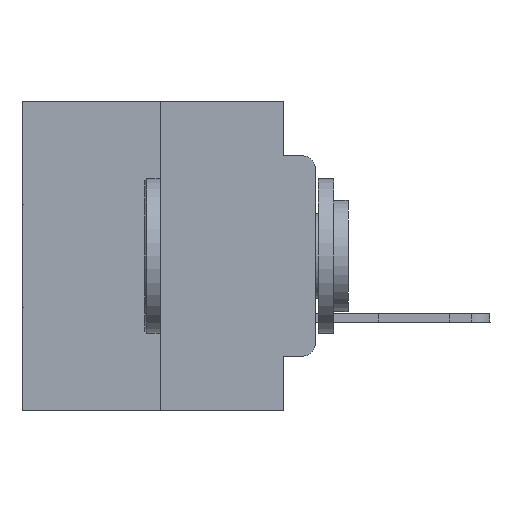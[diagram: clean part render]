
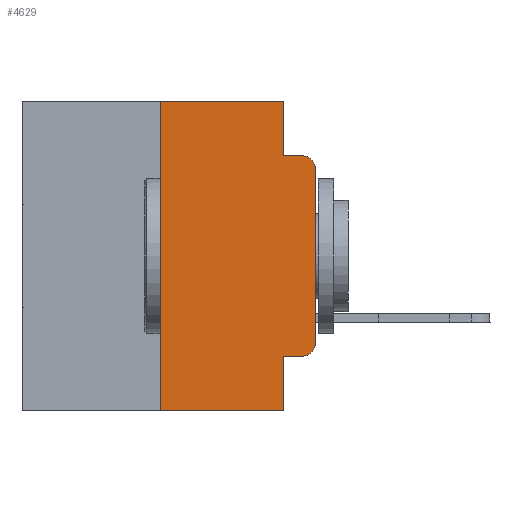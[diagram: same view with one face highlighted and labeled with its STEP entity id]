
A CAD part, left-side view. The second image highlights one B-rep face of the part: STEP entity #4629.
In plain terms, the highlighted planar face has unit normal (-1, 0, 0).
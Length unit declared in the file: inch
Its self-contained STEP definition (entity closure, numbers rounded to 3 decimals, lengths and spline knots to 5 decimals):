
#141 = EDGE_CURVE ( 'NONE', #13487, #4474, #5541, .T. ) ;
#193 = CARTESIAN_POINT ( 'NONE',  ( 0., 0.051, -0.0885 ) ) ;
#568 = CARTESIAN_POINT ( 'NONE',  ( 0., 0.051, 0. ) ) ;
#1051 = CARTESIAN_POINT ( 'NONE',  ( 0., 0.051, -0.4115 ) ) ;
#1135 = FACE_OUTER_BOUND ( 'NONE', #25109, .T. ) ;
#1803 = CARTESIAN_POINT ( 'NONE',  ( 0., 0.051, 0. ) ) ;
#2181 = CARTESIAN_POINT ( 'NONE',  ( 0., 0.02, -0.3915 ) ) ;
#2285 = EDGE_CURVE ( 'NONE', #9579, #4019, #24127, .T. ) ;
#2543 = VECTOR ( 'NONE', #25909, 39.37008 ) ;
#2561 = DIRECTION ( 'NONE',  ( 0., 0., 1. ) ) ;
#2709 = LINE ( 'NONE', #16795, #23457 ) ;
#2901 = DIRECTION ( 'NONE',  ( 0., 0., -1. ) ) ;
#3704 = VERTEX_POINT ( 'NONE', #4943 ) ;
#3713 = VECTOR ( 'NONE', #14315, 39.37008 ) ;
#3853 = CARTESIAN_POINT ( 'NONE',  ( 0., 0.02, -0.1085 ) ) ;
#3874 = CARTESIAN_POINT ( 'NONE',  ( 0., 0.25, -0.5 ) ) ;
#4019 = VERTEX_POINT ( 'NONE', #193 ) ;
#4149 = VERTEX_POINT ( 'NONE', #23626 ) ;
#4474 = VERTEX_POINT ( 'NONE', #25907 ) ;
#4629 = ADVANCED_FACE ( 'NONE', ( #1135 ), #26872, .F. ) ;
#4943 = CARTESIAN_POINT ( 'NONE',  ( 0., 0.051, -0.5 ) ) ;
#5349 = LINE ( 'NONE', #16885, #22020 ) ;
#5541 = LINE ( 'NONE', #1051, #22198 ) ;
#5727 = DIRECTION ( 'NONE',  ( -1., 0., 0. ) ) ;
#6321 = EDGE_CURVE ( 'NONE', #13487, #3704, #18810, .T. ) ;
#6804 = VERTEX_POINT ( 'NONE', #3874 ) ;
#6928 = DIRECTION ( 'NONE',  ( -1., 0., 0. ) ) ;
#7180 = VECTOR ( 'NONE', #21510, 39.37008 ) ;
#8410 = CARTESIAN_POINT ( 'NONE',  ( 0., 0.473, -0.5 ) ) ;
#9579 = VERTEX_POINT ( 'NONE', #568 ) ;
#9618 = LINE ( 'NONE', #27242, #10628 ) ;
#9858 = EDGE_CURVE ( 'NONE', #24876, #9579, #2709, .T. ) ;
#10045 = DIRECTION ( 'NONE',  ( 0., -1., 0. ) ) ;
#10065 = LINE ( 'NONE', #19985, #11460 ) ;
#10079 = AXIS2_PLACEMENT_3D ( 'NONE', #2181, #6928, #13445 ) ;
#10628 = VECTOR ( 'NONE', #18607, 39.37008 ) ;
#11460 = VECTOR ( 'NONE', #2561, 39.37008 ) ;
#11518 = CARTESIAN_POINT ( 'NONE',  ( 0., 0.473, 0. ) ) ;
#12110 = ORIENTED_EDGE ( 'NONE', *, *, #27522, .F. ) ;
#13088 = DIRECTION ( 'NONE',  ( 0., -1., 0. ) ) ;
#13153 = EDGE_CURVE ( 'NONE', #4149, #20485, #19581, .T. ) ;
#13445 = DIRECTION ( 'NONE',  ( 0., 0., -1. ) ) ;
#13487 = VERTEX_POINT ( 'NONE', #20907 ) ;
#14262 = ORIENTED_EDGE ( 'NONE', *, *, #9858, .F. ) ;
#14315 = DIRECTION ( 'NONE',  ( 0., 0., -1. ) ) ;
#14551 = AXIS2_PLACEMENT_3D ( 'NONE', #11518, #24292, #2901 ) ;
#14731 = CARTESIAN_POINT ( 'NONE',  ( 0., 0.02, -0.0885 ) ) ;
#16591 = ORIENTED_EDGE ( 'NONE', *, *, #26675, .T. ) ;
#16795 = CARTESIAN_POINT ( 'NONE',  ( 0., 0.473, 0. ) ) ;
#16858 = CARTESIAN_POINT ( 'NONE',  ( 0., 0.051, 0. ) ) ;
#16885 = CARTESIAN_POINT ( 'NONE',  ( 0., 0., 0. ) ) ;
#17804 = CARTESIAN_POINT ( 'NONE',  ( 0., 0., -0.3915 ) ) ;
#18554 = CARTESIAN_POINT ( 'NONE',  ( 0., 0.25, 0. ) ) ;
#18607 = DIRECTION ( 'NONE',  ( 0., -1., 0. ) ) ;
#18810 = LINE ( 'NONE', #1803, #7180 ) ;
#19470 = EDGE_CURVE ( 'NONE', #4474, #27489, #26313, .T. ) ;
#19581 = CIRCLE ( 'NONE', #27056, 0.02 ) ;
#19985 = CARTESIAN_POINT ( 'NONE',  ( 0., 0.25, 0. ) ) ;
#20100 = EDGE_CURVE ( 'NONE', #4019, #20485, #9618, .T. ) ;
#20353 = ORIENTED_EDGE ( 'NONE', *, *, #6321, .F. ) ;
#20485 = VERTEX_POINT ( 'NONE', #14731 ) ;
#20571 = ORIENTED_EDGE ( 'NONE', *, *, #20100, .F. ) ;
#20907 = CARTESIAN_POINT ( 'NONE',  ( 0., 0.051, -0.4115 ) ) ;
#21384 = ORIENTED_EDGE ( 'NONE', *, *, #141, .T. ) ;
#21510 = DIRECTION ( 'NONE',  ( 0., 0., -1. ) ) ;
#22020 = VECTOR ( 'NONE', #26059, 39.37008 ) ;
#22198 = VECTOR ( 'NONE', #10045, 39.37008 ) ;
#22902 = ORIENTED_EDGE ( 'NONE', *, *, #2285, .F. ) ;
#23457 = VECTOR ( 'NONE', #13088, 39.37008 ) ;
#23626 = CARTESIAN_POINT ( 'NONE',  ( 0., 0., -0.1085 ) ) ;
#24127 = LINE ( 'NONE', #16858, #3713 ) ;
#24231 = ORIENTED_EDGE ( 'NONE', *, *, #25123, .T. ) ;
#24292 = DIRECTION ( 'NONE',  ( 1., 0., 0. ) ) ;
#24557 = ORIENTED_EDGE ( 'NONE', *, *, #19470, .T. ) ;
#24876 = VERTEX_POINT ( 'NONE', #18554 ) ;
#25109 = EDGE_LOOP ( 'NONE', ( #24231, #26506, #20571, #22902, #14262, #12110, #16591, #20353, #21384, #24557 ) ) ;
#25123 = EDGE_CURVE ( 'NONE', #27489, #4149, #5349, .T. ) ;
#25907 = CARTESIAN_POINT ( 'NONE',  ( 0., 0.02, -0.4115 ) ) ;
#25909 = DIRECTION ( 'NONE',  ( 0., -1., 0. ) ) ;
#26059 = DIRECTION ( 'NONE',  ( 0., 0., 1. ) ) ;
#26313 = CIRCLE ( 'NONE', #10079, 0.02 ) ;
#26383 = LINE ( 'NONE', #8410, #2543 ) ;
#26506 = ORIENTED_EDGE ( 'NONE', *, *, #13153, .T. ) ;
#26675 = EDGE_CURVE ( 'NONE', #6804, #3704, #26383, .T. ) ;
#26872 = PLANE ( 'NONE',  #14551 ) ;
#27056 = AXIS2_PLACEMENT_3D ( 'NONE', #3853, #5727, #27725 ) ;
#27242 = CARTESIAN_POINT ( 'NONE',  ( 0., 0.051, -0.0885 ) ) ;
#27489 = VERTEX_POINT ( 'NONE', #17804 ) ;
#27522 = EDGE_CURVE ( 'NONE', #6804, #24876, #10065, .T. ) ;
#27725 = DIRECTION ( 'NONE',  ( 0., 0., -1. ) ) ;
